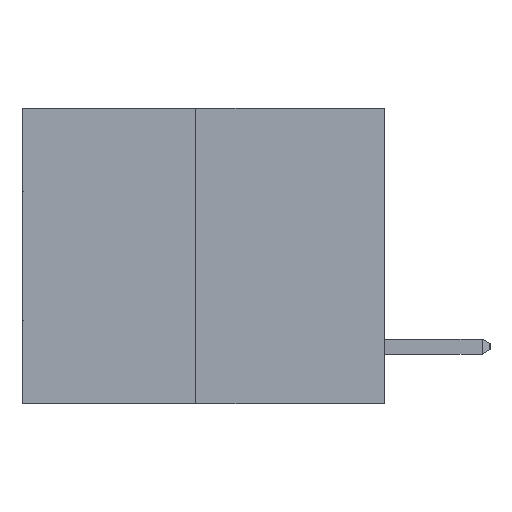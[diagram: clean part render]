
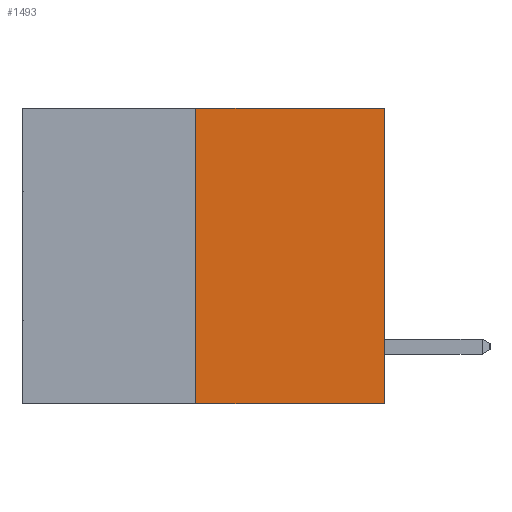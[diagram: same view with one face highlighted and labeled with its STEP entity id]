
A CAD part, left-side view. The second image highlights one B-rep face of the part: STEP entity #1493.
In plain terms, the highlighted planar face has unit normal (-1, 0, 0).
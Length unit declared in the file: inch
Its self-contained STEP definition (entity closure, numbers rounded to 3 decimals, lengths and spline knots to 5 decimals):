
#50 = VECTOR ( 'NONE', #7285, 39.37008 ) ;
#877 = CARTESIAN_POINT ( 'NONE',  ( 0., 0.6, 0. ) ) ;
#1493 = ADVANCED_FACE ( 'NONE', ( #21183 ), #22104, .F. ) ;
#2713 = CARTESIAN_POINT ( 'NONE',  ( 0., 0.6, -0.49 ) ) ;
#3233 = EDGE_CURVE ( 'NONE', #29800, #19452, #3652, .T. ) ;
#3652 = LINE ( 'NONE', #30671, #21794 ) ;
#3778 = LINE ( 'NONE', #4912, #50 ) ;
#4912 = CARTESIAN_POINT ( 'NONE',  ( 0., 0., 0. ) ) ;
#6452 = EDGE_LOOP ( 'NONE', ( #18481, #15669, #22452, #24576 ) ) ;
#7285 = DIRECTION ( 'NONE',  ( 0., 0., 1. ) ) ;
#8869 = CARTESIAN_POINT ( 'NONE',  ( 0., 0., -0.49 ) ) ;
#10411 = VERTEX_POINT ( 'NONE', #8869 ) ;
#11023 = EDGE_CURVE ( 'NONE', #29800, #10411, #28203, .T. ) ;
#11619 = LINE ( 'NONE', #29995, #18658 ) ;
#14521 = DIRECTION ( 'NONE',  ( 0., -1., 0. ) ) ;
#15669 = ORIENTED_EDGE ( 'NONE', *, *, #11023, .T. ) ;
#15757 = DIRECTION ( 'NONE',  ( 0., -1., 0. ) ) ;
#16470 = DIRECTION ( 'NONE',  ( 0., 0., 1. ) ) ;
#18481 = ORIENTED_EDGE ( 'NONE', *, *, #3233, .F. ) ;
#18585 = CARTESIAN_POINT ( 'NONE',  ( 0., 0.312, 0. ) ) ;
#18658 = VECTOR ( 'NONE', #15757, 39.37008 ) ;
#19452 = VERTEX_POINT ( 'NONE', #18585 ) ;
#19826 = DIRECTION ( 'NONE',  ( 0., 0., -1. ) ) ;
#19866 = EDGE_CURVE ( 'NONE', #10411, #21358, #3778, .T. ) ;
#21183 = FACE_OUTER_BOUND ( 'NONE', #6452, .T. ) ;
#21358 = VERTEX_POINT ( 'NONE', #22326 ) ;
#21794 = VECTOR ( 'NONE', #16470, 39.37008 ) ;
#22104 = PLANE ( 'NONE',  #29322 ) ;
#22326 = CARTESIAN_POINT ( 'NONE',  ( 0., 0., 0. ) ) ;
#22452 = ORIENTED_EDGE ( 'NONE', *, *, #19866, .T. ) ;
#24466 = CARTESIAN_POINT ( 'NONE',  ( 0., 0.312, -0.49 ) ) ;
#24576 = ORIENTED_EDGE ( 'NONE', *, *, #30533, .F. ) ;
#28203 = LINE ( 'NONE', #2713, #28961 ) ;
#28961 = VECTOR ( 'NONE', #14521, 39.37008 ) ;
#29322 = AXIS2_PLACEMENT_3D ( 'NONE', #877, #29530, #19826 ) ;
#29530 = DIRECTION ( 'NONE',  ( 1., 0., 0. ) ) ;
#29800 = VERTEX_POINT ( 'NONE', #24466 ) ;
#29995 = CARTESIAN_POINT ( 'NONE',  ( 0., 0.6, 0. ) ) ;
#30533 = EDGE_CURVE ( 'NONE', #19452, #21358, #11619, .T. ) ;
#30671 = CARTESIAN_POINT ( 'NONE',  ( 0., 0.312, -0.49 ) ) ;
